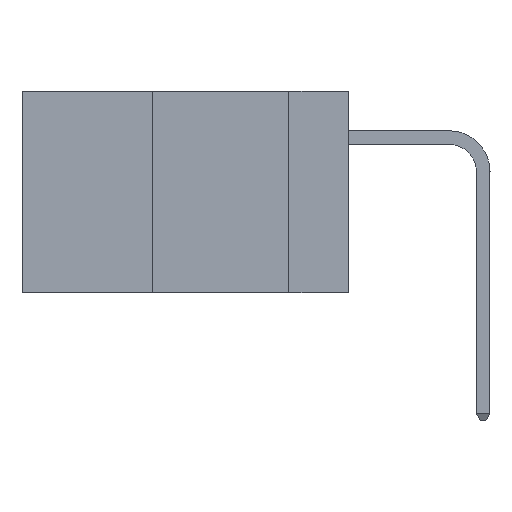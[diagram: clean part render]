
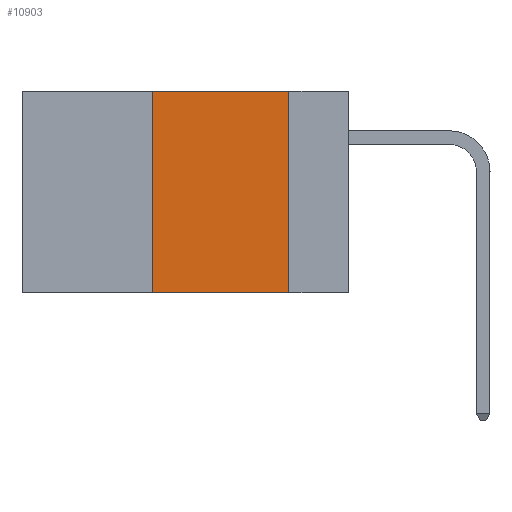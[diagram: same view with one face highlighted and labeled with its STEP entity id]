
A CAD part, left-side view. The second image highlights one B-rep face of the part: STEP entity #10903.
In plain terms, the highlighted planar face has unit normal (-1, 0, 0).
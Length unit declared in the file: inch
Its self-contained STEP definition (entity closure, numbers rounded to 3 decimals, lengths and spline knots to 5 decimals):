
#567 = LINE ( 'NONE', #10940, #6402 ) ;
#766 = CARTESIAN_POINT ( 'NONE',  ( 0., 0.11, -0.37 ) ) ;
#785 = VECTOR ( 'NONE', #5367, 39.37008 ) ;
#1319 = DIRECTION ( 'NONE',  ( 1., 0., 0. ) ) ;
#1323 = CARTESIAN_POINT ( 'NONE',  ( 0., 0.36, -0.37 ) ) ;
#1524 = DIRECTION ( 'NONE',  ( 0., -1., 0. ) ) ;
#2705 = DIRECTION ( 'NONE',  ( 0., 0., 1. ) ) ;
#3015 = CARTESIAN_POINT ( 'NONE',  ( 0., 0.11, 0. ) ) ;
#3122 = DIRECTION ( 'NONE',  ( 0., 0., -1. ) ) ;
#3184 = ORIENTED_EDGE ( 'NONE', *, *, #5994, .F. ) ;
#3271 = EDGE_LOOP ( 'NONE', ( #3184, #7586, #4491, #9225 ) ) ;
#4091 = DIRECTION ( 'NONE',  ( 0., -1., 0. ) ) ;
#4454 = CARTESIAN_POINT ( 'NONE',  ( 0., 0.11, 0. ) ) ;
#4491 = ORIENTED_EDGE ( 'NONE', *, *, #8958, .F. ) ;
#5150 = CARTESIAN_POINT ( 'NONE',  ( 0., 0.36, 0. ) ) ;
#5208 = CARTESIAN_POINT ( 'NONE',  ( 0., 0.6, -0.37 ) ) ;
#5241 = FACE_OUTER_BOUND ( 'NONE', #3271, .T. ) ;
#5367 = DIRECTION ( 'NONE',  ( 0., 0., -1. ) ) ;
#5994 = EDGE_CURVE ( 'NONE', #9253, #8071, #8223, .T. ) ;
#6185 = VECTOR ( 'NONE', #1524, 39.37008 ) ;
#6187 = EDGE_CURVE ( 'NONE', #7162, #8071, #10986, .T. ) ;
#6402 = VECTOR ( 'NONE', #4091, 39.37008 ) ;
#6759 = CARTESIAN_POINT ( 'NONE',  ( 0., 0.36, 0. ) ) ;
#7162 = VERTEX_POINT ( 'NONE', #1323 ) ;
#7346 = VECTOR ( 'NONE', #2705, 39.37008 ) ;
#7586 = ORIENTED_EDGE ( 'NONE', *, *, #8523, .F. ) ;
#8071 = VERTEX_POINT ( 'NONE', #766 ) ;
#8223 = LINE ( 'NONE', #4454, #785 ) ;
#8428 = LINE ( 'NONE', #5150, #7346 ) ;
#8523 = EDGE_CURVE ( 'NONE', #10625, #9253, #567, .T. ) ;
#8942 = AXIS2_PLACEMENT_3D ( 'NONE', #10084, #1319, #3122 ) ;
#8958 = EDGE_CURVE ( 'NONE', #7162, #10625, #8428, .T. ) ;
#9195 = PLANE ( 'NONE',  #8942 ) ;
#9225 = ORIENTED_EDGE ( 'NONE', *, *, #6187, .T. ) ;
#9253 = VERTEX_POINT ( 'NONE', #3015 ) ;
#10084 = CARTESIAN_POINT ( 'NONE',  ( 0., 0.6, 0. ) ) ;
#10625 = VERTEX_POINT ( 'NONE', #6759 ) ;
#10903 = ADVANCED_FACE ( 'NONE', ( #5241 ), #9195, .F. ) ;
#10940 = CARTESIAN_POINT ( 'NONE',  ( 0., 0.6, 0. ) ) ;
#10986 = LINE ( 'NONE', #5208, #6185 ) ;
